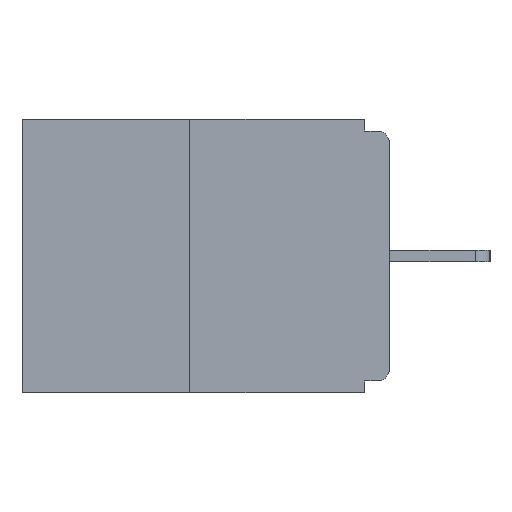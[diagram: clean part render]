
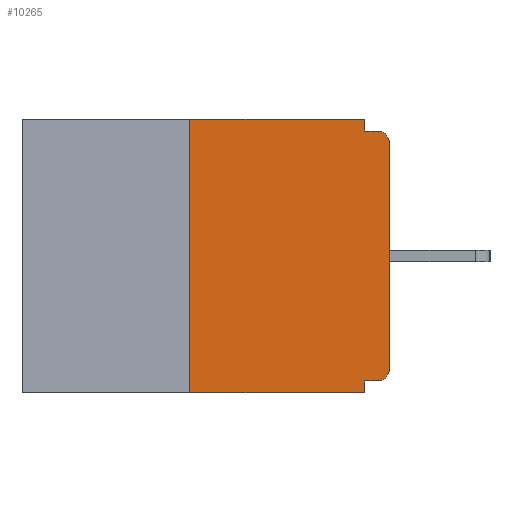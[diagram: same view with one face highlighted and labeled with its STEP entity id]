
A CAD part, left-side view. The second image highlights one B-rep face of the part: STEP entity #10265.
In plain terms, the highlighted planar face has unit normal (-1, 0, 0).
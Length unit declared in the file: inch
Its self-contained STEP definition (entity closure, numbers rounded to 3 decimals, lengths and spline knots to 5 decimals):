
#160 = CARTESIAN_POINT ( 'NONE',  ( 0., 0.015, -0.328 ) ) ;
#276 = DIRECTION ( 'NONE',  ( 0., -1., 0. ) ) ;
#599 = VERTEX_POINT ( 'NONE', #10765 ) ;
#859 = EDGE_CURVE ( 'NONE', #896, #18212, #16109, .T. ) ;
#874 = CARTESIAN_POINT ( 'NONE',  ( 0., 0.25, 0. ) ) ;
#896 = VERTEX_POINT ( 'NONE', #18373 ) ;
#1082 = CARTESIAN_POINT ( 'NONE',  ( 0., 0.25, 0. ) ) ;
#1287 = VECTOR ( 'NONE', #9630, 39.37008 ) ;
#1695 = LINE ( 'NONE', #7748, #8441 ) ;
#2031 = EDGE_CURVE ( 'NONE', #15530, #16191, #7456, .T. ) ;
#2102 = DIRECTION ( 'NONE',  ( 0., 0., -1. ) ) ;
#2539 = LINE ( 'NONE', #15769, #1287 ) ;
#2889 = ORIENTED_EDGE ( 'NONE', *, *, #12337, .T. ) ;
#3259 = ORIENTED_EDGE ( 'NONE', *, *, #11989, .T. ) ;
#3361 = DIRECTION ( 'NONE',  ( 0., 0., -1. ) ) ;
#3969 = VERTEX_POINT ( 'NONE', #1082 ) ;
#4028 = CARTESIAN_POINT ( 'NONE',  ( 0., 0.46, -0.343 ) ) ;
#4166 = EDGE_LOOP ( 'NONE', ( #12191, #14737, #11616, #8293, #11040, #3259, #2889, #6852, #12424, #4948 ) ) ;
#4209 = VERTEX_POINT ( 'NONE', #17602 ) ;
#4567 = VECTOR ( 'NONE', #12281, 39.37008 ) ;
#4578 = DIRECTION ( 'NONE',  ( -1., 0., 0. ) ) ;
#4709 = VERTEX_POINT ( 'NONE', #7569 ) ;
#4948 = ORIENTED_EDGE ( 'NONE', *, *, #859, .F. ) ;
#4977 = VERTEX_POINT ( 'NONE', #17377 ) ;
#5211 = DIRECTION ( 'NONE',  ( 0., 0., 1. ) ) ;
#5363 = VECTOR ( 'NONE', #5211, 39.37008 ) ;
#5798 = CIRCLE ( 'NONE', #18454, 0.015 ) ;
#6414 = LINE ( 'NONE', #12258, #14517 ) ;
#6530 = CARTESIAN_POINT ( 'NONE',  ( 0., 0., 0. ) ) ;
#6544 = EDGE_CURVE ( 'NONE', #599, #3969, #6733, .T. ) ;
#6552 = CARTESIAN_POINT ( 'NONE',  ( 0., 0.015, -0.313 ) ) ;
#6733 = LINE ( 'NONE', #874, #5363 ) ;
#6790 = CARTESIAN_POINT ( 'NONE',  ( 0., 0.031, -0.015 ) ) ;
#6852 = ORIENTED_EDGE ( 'NONE', *, *, #15652, .T. ) ;
#7456 = LINE ( 'NONE', #8961, #13122 ) ;
#7569 = CARTESIAN_POINT ( 'NONE',  ( 0., 0.031, -0.343 ) ) ;
#7581 = AXIS2_PLACEMENT_3D ( 'NONE', #15070, #13661, #11774 ) ;
#7748 = CARTESIAN_POINT ( 'NONE',  ( 0., 0.46, 0. ) ) ;
#8293 = ORIENTED_EDGE ( 'NONE', *, *, #10897, .F. ) ;
#8441 = VECTOR ( 'NONE', #276, 39.37008 ) ;
#8933 = CARTESIAN_POINT ( 'NONE',  ( 0., 0.031, 0. ) ) ;
#8961 = CARTESIAN_POINT ( 'NONE',  ( 0., 0., -0.328 ) ) ;
#9314 = PLANE ( 'NONE',  #7581 ) ;
#9630 = DIRECTION ( 'NONE',  ( 0., -1., 0. ) ) ;
#9999 = CIRCLE ( 'NONE', #11193, 0.015 ) ;
#10265 = ADVANCED_FACE ( 'NONE', ( #12160 ), #9314, .F. ) ;
#10511 = VECTOR ( 'NONE', #3361, 39.37008 ) ;
#10638 = DIRECTION ( 'NONE',  ( 0., 0., -1. ) ) ;
#10765 = CARTESIAN_POINT ( 'NONE',  ( 0., 0.25, -0.343 ) ) ;
#10897 = EDGE_CURVE ( 'NONE', #16191, #4709, #6414, .T. ) ;
#11028 = EDGE_CURVE ( 'NONE', #599, #4709, #14037, .T. ) ;
#11040 = ORIENTED_EDGE ( 'NONE', *, *, #2031, .F. ) ;
#11193 = AXIS2_PLACEMENT_3D ( 'NONE', #6552, #12489, #2102 ) ;
#11616 = ORIENTED_EDGE ( 'NONE', *, *, #11028, .T. ) ;
#11774 = DIRECTION ( 'NONE',  ( 0., 0., -1. ) ) ;
#11978 = DIRECTION ( 'NONE',  ( 0., 1., 0. ) ) ;
#11989 = EDGE_CURVE ( 'NONE', #15530, #13403, #9999, .T. ) ;
#12160 = FACE_OUTER_BOUND ( 'NONE', #4166, .T. ) ;
#12191 = ORIENTED_EDGE ( 'NONE', *, *, #13905, .F. ) ;
#12258 = CARTESIAN_POINT ( 'NONE',  ( 0., 0.031, -0.343 ) ) ;
#12281 = DIRECTION ( 'NONE',  ( 0., 0., 1. ) ) ;
#12337 = EDGE_CURVE ( 'NONE', #13403, #4977, #13875, .T. ) ;
#12424 = ORIENTED_EDGE ( 'NONE', *, *, #17875, .F. ) ;
#12489 = DIRECTION ( 'NONE',  ( -1., 0., 0. ) ) ;
#13122 = VECTOR ( 'NONE', #11978, 39.37008 ) ;
#13403 = VERTEX_POINT ( 'NONE', #16369 ) ;
#13523 = CARTESIAN_POINT ( 'NONE',  ( 0., 0.031, -0.328 ) ) ;
#13661 = DIRECTION ( 'NONE',  ( 1., 0., 0. ) ) ;
#13875 = LINE ( 'NONE', #6530, #4567 ) ;
#13905 = EDGE_CURVE ( 'NONE', #3969, #896, #1695, .T. ) ;
#14037 = LINE ( 'NONE', #4028, #16595 ) ;
#14517 = VECTOR ( 'NONE', #14901, 39.37008 ) ;
#14737 = ORIENTED_EDGE ( 'NONE', *, *, #6544, .F. ) ;
#14901 = DIRECTION ( 'NONE',  ( 0., 0., -1. ) ) ;
#15070 = CARTESIAN_POINT ( 'NONE',  ( 0., 0.46, 0. ) ) ;
#15530 = VERTEX_POINT ( 'NONE', #160 ) ;
#15652 = EDGE_CURVE ( 'NONE', #4977, #4209, #5798, .T. ) ;
#15769 = CARTESIAN_POINT ( 'NONE',  ( 0., 0., -0.015 ) ) ;
#16109 = LINE ( 'NONE', #8933, #10511 ) ;
#16191 = VERTEX_POINT ( 'NONE', #13523 ) ;
#16369 = CARTESIAN_POINT ( 'NONE',  ( 0., 0., -0.313 ) ) ;
#16595 = VECTOR ( 'NONE', #16690, 39.37008 ) ;
#16690 = DIRECTION ( 'NONE',  ( 0., -1., 0. ) ) ;
#17377 = CARTESIAN_POINT ( 'NONE',  ( 0., 0., -0.03 ) ) ;
#17602 = CARTESIAN_POINT ( 'NONE',  ( 0., 0.015, -0.015 ) ) ;
#17714 = CARTESIAN_POINT ( 'NONE',  ( 0., 0.015, -0.03 ) ) ;
#17875 = EDGE_CURVE ( 'NONE', #18212, #4209, #2539, .T. ) ;
#18212 = VERTEX_POINT ( 'NONE', #6790 ) ;
#18373 = CARTESIAN_POINT ( 'NONE',  ( 0., 0.031, 0. ) ) ;
#18454 = AXIS2_PLACEMENT_3D ( 'NONE', #17714, #4578, #10638 ) ;
